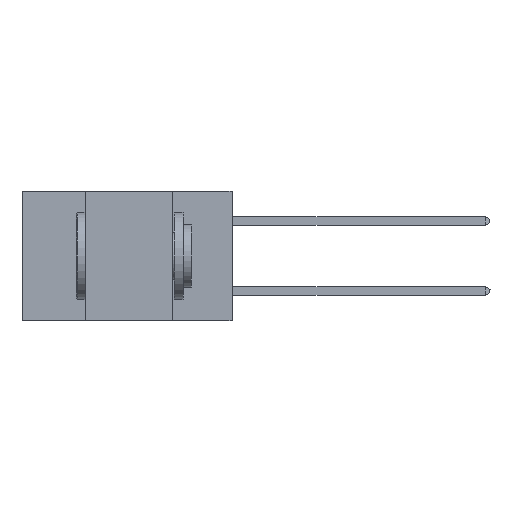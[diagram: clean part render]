
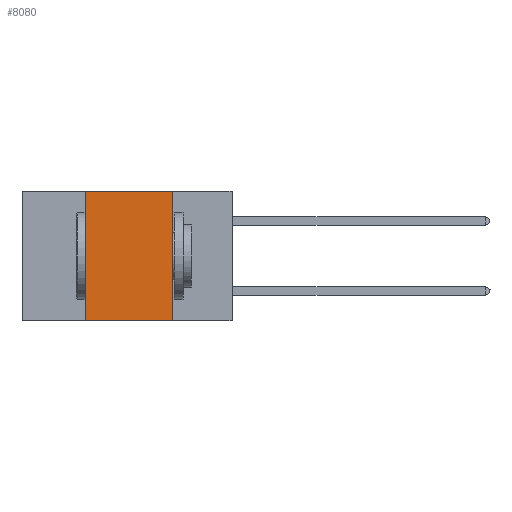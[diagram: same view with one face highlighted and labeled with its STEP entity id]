
A CAD part, left-side view. The second image highlights one B-rep face of the part: STEP entity #8080.
In plain terms, the highlighted planar face has unit normal (-1, 0, 0).
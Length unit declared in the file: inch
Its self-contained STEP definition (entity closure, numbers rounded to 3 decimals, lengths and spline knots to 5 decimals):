
#264 = FACE_OUTER_BOUND ( 'NONE', #1997, .T. ) ;
#430 = CARTESIAN_POINT ( 'NONE',  ( 0., 0.42, 0. ) ) ;
#1315 = DIRECTION ( 'NONE',  ( 1., 0., 0. ) ) ;
#1595 = VERTEX_POINT ( 'NONE', #5059 ) ;
#1895 = DIRECTION ( 'NONE',  ( 0., 0., 1. ) ) ;
#1997 = EDGE_LOOP ( 'NONE', ( #9267, #3215, #9994, #8524 ) ) ;
#3215 = ORIENTED_EDGE ( 'NONE', *, *, #4598, .F. ) ;
#3485 = VERTEX_POINT ( 'NONE', #5890 ) ;
#4570 = CARTESIAN_POINT ( 'NONE',  ( 0., 0.42, -0.37 ) ) ;
#4598 = EDGE_CURVE ( 'NONE', #3485, #6152, #10333, .T. ) ;
#5059 = CARTESIAN_POINT ( 'NONE',  ( 0., 0.17, -0.37 ) ) ;
#5303 = CARTESIAN_POINT ( 'NONE',  ( 0., 0.17, 0. ) ) ;
#5890 = CARTESIAN_POINT ( 'NONE',  ( 0., 0.42, 0. ) ) ;
#5957 = EDGE_CURVE ( 'NONE', #7544, #3485, #17900, .T. ) ;
#6152 = VERTEX_POINT ( 'NONE', #5303 ) ;
#6919 = CARTESIAN_POINT ( 'NONE',  ( 0., 0.6, -0.37 ) ) ;
#7153 = CARTESIAN_POINT ( 'NONE',  ( 0., 0.17, 0. ) ) ;
#7544 = VERTEX_POINT ( 'NONE', #4570 ) ;
#7555 = CARTESIAN_POINT ( 'NONE',  ( 0., 0.6, 0. ) ) ;
#8080 = ADVANCED_FACE ( 'NONE', ( #264 ), #9988, .F. ) ;
#8524 = ORIENTED_EDGE ( 'NONE', *, *, #13844, .T. ) ;
#8770 = VECTOR ( 'NONE', #11409, 39.37008 ) ;
#9267 = ORIENTED_EDGE ( 'NONE', *, *, #12588, .F. ) ;
#9988 = PLANE ( 'NONE',  #14284 ) ;
#9994 = ORIENTED_EDGE ( 'NONE', *, *, #5957, .F. ) ;
#10333 = LINE ( 'NONE', #7555, #10776 ) ;
#10728 = VECTOR ( 'NONE', #1895, 39.37008 ) ;
#10776 = VECTOR ( 'NONE', #17148, 39.37008 ) ;
#10973 = LINE ( 'NONE', #6919, #14181 ) ;
#11405 = DIRECTION ( 'NONE',  ( 0., 0., -1. ) ) ;
#11409 = DIRECTION ( 'NONE',  ( 0., 0., -1. ) ) ;
#12525 = LINE ( 'NONE', #7153, #8770 ) ;
#12588 = EDGE_CURVE ( 'NONE', #6152, #1595, #12525, .T. ) ;
#12729 = CARTESIAN_POINT ( 'NONE',  ( 0., 0.6, 0. ) ) ;
#13844 = EDGE_CURVE ( 'NONE', #7544, #1595, #10973, .T. ) ;
#14181 = VECTOR ( 'NONE', #16679, 39.37008 ) ;
#14284 = AXIS2_PLACEMENT_3D ( 'NONE', #12729, #1315, #11405 ) ;
#16679 = DIRECTION ( 'NONE',  ( 0., -1., 0. ) ) ;
#17148 = DIRECTION ( 'NONE',  ( 0., -1., 0. ) ) ;
#17900 = LINE ( 'NONE', #430, #10728 ) ;
